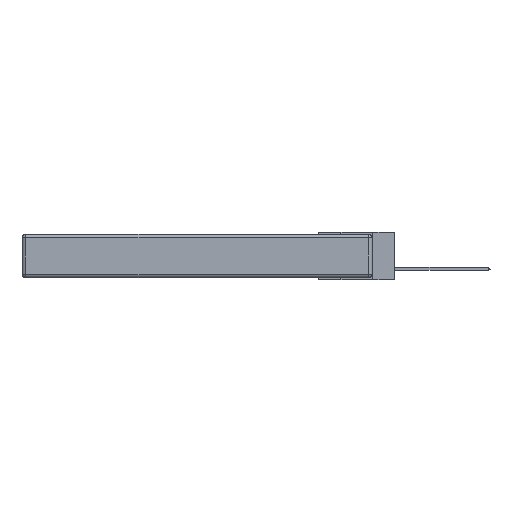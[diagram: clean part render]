
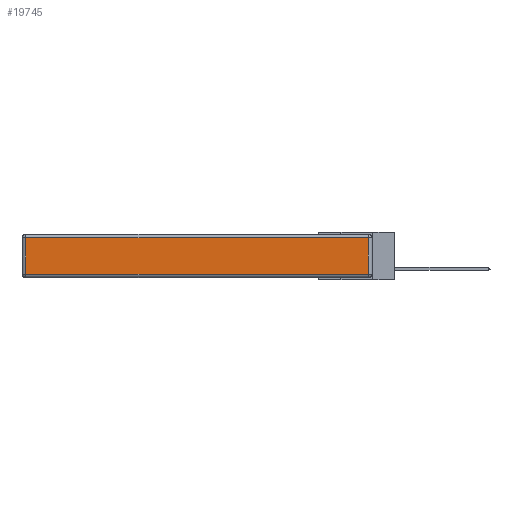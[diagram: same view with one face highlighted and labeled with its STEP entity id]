
A CAD part, left-side view. The second image highlights one B-rep face of the part: STEP entity #19745.
In plain terms, the highlighted planar face has unit normal (-1, 0, 0).
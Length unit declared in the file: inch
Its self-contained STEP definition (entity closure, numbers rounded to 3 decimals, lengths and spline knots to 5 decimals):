
#1454 = PLANE ( 'NONE',  #19870 ) ;
#2633 = LINE ( 'NONE', #15955, #10746 ) ;
#2867 = EDGE_CURVE ( 'NONE', #22369, #11776, #22614, .T. ) ;
#3131 = CARTESIAN_POINT ( 'NONE',  ( 0., 2.72, -0.343 ) ) ;
#3190 = CARTESIAN_POINT ( 'NONE',  ( 0., 0., -0.343 ) ) ;
#3278 = DIRECTION ( 'NONE',  ( 0., 0., 1. ) ) ;
#6156 = CARTESIAN_POINT ( 'NONE',  ( 0., 2.72, -0.03 ) ) ;
#6599 = ORIENTED_EDGE ( 'NONE', *, *, #2867, .T. ) ;
#7437 = EDGE_CURVE ( 'NONE', #11305, #22369, #18356, .T. ) ;
#7478 = DIRECTION ( 'NONE',  ( 0., 1., 0. ) ) ;
#7705 = LINE ( 'NONE', #12769, #14711 ) ;
#8030 = ORIENTED_EDGE ( 'NONE', *, *, #8859, .T. ) ;
#8111 = EDGE_CURVE ( 'NONE', #22690, #11305, #7705, .T. ) ;
#8857 = CARTESIAN_POINT ( 'NONE',  ( 0., 2.72, -0.313 ) ) ;
#8859 = EDGE_CURVE ( 'NONE', #11776, #22690, #2633, .T. ) ;
#9200 = CARTESIAN_POINT ( 'NONE',  ( 0., 0.03, -0.313 ) ) ;
#9261 = DIRECTION ( 'NONE',  ( 0., 0., 1. ) ) ;
#9691 = VECTOR ( 'NONE', #7478, 39.37008 ) ;
#10603 = EDGE_LOOP ( 'NONE', ( #8030, #19984, #15018, #6599 ) ) ;
#10746 = VECTOR ( 'NONE', #22997, 39.37008 ) ;
#11305 = VERTEX_POINT ( 'NONE', #20986 ) ;
#11776 = VERTEX_POINT ( 'NONE', #8857 ) ;
#12769 = CARTESIAN_POINT ( 'NONE',  ( 0., 0.03, -0.343 ) ) ;
#13963 = DIRECTION ( 'NONE',  ( -1., 0., 0. ) ) ;
#14303 = VECTOR ( 'NONE', #15474, 39.37008 ) ;
#14711 = VECTOR ( 'NONE', #9261, 39.37008 ) ;
#15018 = ORIENTED_EDGE ( 'NONE', *, *, #7437, .T. ) ;
#15474 = DIRECTION ( 'NONE',  ( 0., 0., -1. ) ) ;
#15955 = CARTESIAN_POINT ( 'NONE',  ( 0., 0., -0.313 ) ) ;
#17450 = CARTESIAN_POINT ( 'NONE',  ( 0., 2.75, -0.03 ) ) ;
#18356 = LINE ( 'NONE', #17450, #9691 ) ;
#19745 = ADVANCED_FACE ( 'NONE', ( #21762 ), #1454, .T. ) ;
#19870 = AXIS2_PLACEMENT_3D ( 'NONE', #3190, #13963, #3278 ) ;
#19984 = ORIENTED_EDGE ( 'NONE', *, *, #8111, .T. ) ;
#20986 = CARTESIAN_POINT ( 'NONE',  ( 0., 0.03, -0.03 ) ) ;
#21762 = FACE_OUTER_BOUND ( 'NONE', #10603, .T. ) ;
#22369 = VERTEX_POINT ( 'NONE', #6156 ) ;
#22614 = LINE ( 'NONE', #3131, #14303 ) ;
#22690 = VERTEX_POINT ( 'NONE', #9200 ) ;
#22997 = DIRECTION ( 'NONE',  ( 0., -1., 0. ) ) ;
